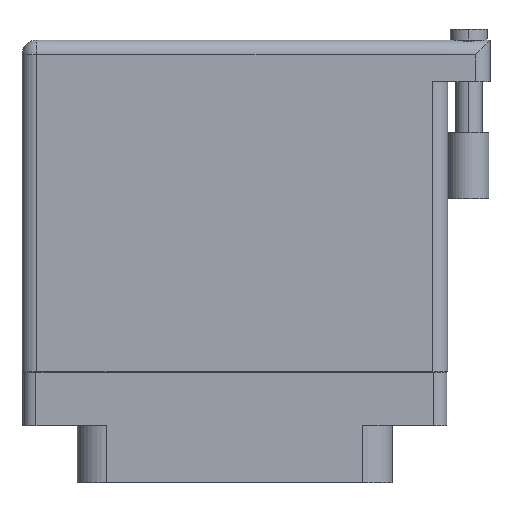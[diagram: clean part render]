
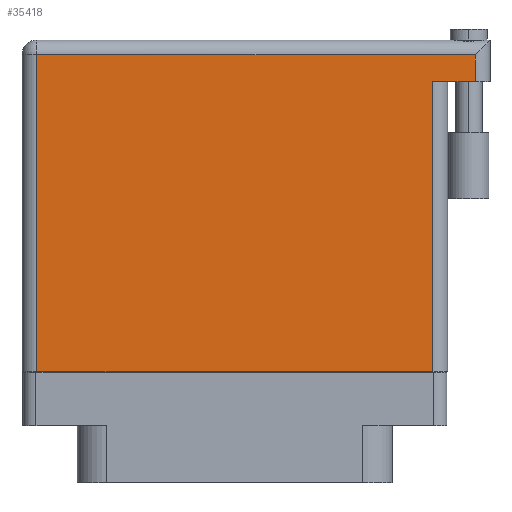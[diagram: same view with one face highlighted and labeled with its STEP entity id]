
A CAD part, front view. The second image highlights one B-rep face of the part: STEP entity #35418.
In plain terms, the highlighted face is planar.
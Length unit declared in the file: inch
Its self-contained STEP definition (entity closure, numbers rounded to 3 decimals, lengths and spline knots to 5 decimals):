
#506 = EDGE_CURVE ( 'NONE', #37140, #34961, #4797, .T. ) ;
#1290 = EDGE_CURVE ( 'NONE', #16771, #7316, #10068, .T. ) ;
#1339 = LINE ( 'NONE', #14774, #28770 ) ;
#1908 = CARTESIAN_POINT ( 'NONE',  ( 0.934, 1.269, 0.4495 ) ) ;
#2049 = DIRECTION ( 'NONE',  ( -1., 0., 0. ) ) ;
#2060 = EDGE_CURVE ( 'NONE', #34961, #11494, #1339, .T. ) ;
#2400 = PLANE ( 'NONE',  #3954 ) ;
#2405 = DIRECTION ( 'NONE',  ( 0., -1., 0. ) ) ;
#3937 = VECTOR ( 'NONE', #26450, 39.37008 ) ;
#3954 = AXIS2_PLACEMENT_3D ( 'NONE', #21040, #33476, #18112 ) ;
#4003 = CARTESIAN_POINT ( 'NONE',  ( 1.134, 1.466, 0.4495 ) ) ;
#4797 = LINE ( 'NONE', #32863, #17341 ) ;
#5541 = EDGE_CURVE ( 'NONE', #11494, #21737, #5852, .T. ) ;
#5654 = ORIENTED_EDGE ( 'NONE', *, *, #12906, .T. ) ;
#5807 = EDGE_LOOP ( 'NONE', ( #34716, #5654, #22525, #21060, #19671, #14708 ) ) ;
#5836 = DIRECTION ( 'NONE',  ( 1., 0., 0. ) ) ;
#5852 = LINE ( 'NONE', #18614, #23176 ) ;
#6847 = CARTESIAN_POINT ( 'NONE',  ( 0.934, -0.1, 0.4495 ) ) ;
#7316 = VERTEX_POINT ( 'NONE', #39706 ) ;
#7902 = FACE_OUTER_BOUND ( 'NONE', #5807, .T. ) ;
#9822 = DIRECTION ( 'NONE',  ( -1., 0., 0. ) ) ;
#10068 = LINE ( 'NONE', #12647, #31269 ) ;
#11494 = VERTEX_POINT ( 'NONE', #35452 ) ;
#12647 = CARTESIAN_POINT ( 'NONE',  ( 1.204, 1.269, 0.4495 ) ) ;
#12906 = EDGE_CURVE ( 'NONE', #21737, #7316, #27032, .T. ) ;
#13142 = LINE ( 'NONE', #4003, #30462 ) ;
#14708 = ORIENTED_EDGE ( 'NONE', *, *, #2060, .T. ) ;
#14774 = CARTESIAN_POINT ( 'NONE',  ( -0.934, -0.1, 0.4495 ) ) ;
#15809 = CARTESIAN_POINT ( 'NONE',  ( 1.134, 1.269, 0.4495 ) ) ;
#16771 = VERTEX_POINT ( 'NONE', #15809 ) ;
#17341 = VECTOR ( 'NONE', #2049, 39.37008 ) ;
#18112 = DIRECTION ( 'NONE',  ( -1., 0., 0. ) ) ;
#18614 = CARTESIAN_POINT ( 'NONE',  ( -1.004, -0.1, 0.4495 ) ) ;
#19198 = DIRECTION ( 'NONE',  ( 0., 1., 0. ) ) ;
#19671 = ORIENTED_EDGE ( 'NONE', *, *, #506, .T. ) ;
#21040 = CARTESIAN_POINT ( 'NONE',  ( -1.004, 1.466, 0.4495 ) ) ;
#21060 = ORIENTED_EDGE ( 'NONE', *, *, #26642, .T. ) ;
#21737 = VERTEX_POINT ( 'NONE', #6847 ) ;
#22280 = CARTESIAN_POINT ( 'NONE',  ( -0.934, 1.396, 0.4495 ) ) ;
#22525 = ORIENTED_EDGE ( 'NONE', *, *, #1290, .F. ) ;
#23176 = VECTOR ( 'NONE', #5836, 39.37008 ) ;
#25771 = CARTESIAN_POINT ( 'NONE',  ( 1.134, 1.396, 0.4495 ) ) ;
#26450 = DIRECTION ( 'NONE',  ( 0., 1., 0. ) ) ;
#26642 = EDGE_CURVE ( 'NONE', #16771, #37140, #13142, .T. ) ;
#27032 = LINE ( 'NONE', #1908, #3937 ) ;
#28770 = VECTOR ( 'NONE', #2405, 39.37008 ) ;
#30462 = VECTOR ( 'NONE', #19198, 39.37008 ) ;
#31269 = VECTOR ( 'NONE', #9822, 39.37008 ) ;
#32863 = CARTESIAN_POINT ( 'NONE',  ( -1.004, 1.396, 0.4495 ) ) ;
#33476 = DIRECTION ( 'NONE',  ( 0., 0., -1. ) ) ;
#34716 = ORIENTED_EDGE ( 'NONE', *, *, #5541, .T. ) ;
#34961 = VERTEX_POINT ( 'NONE', #22280 ) ;
#35418 = ADVANCED_FACE ( 'NONE', ( #7902 ), #2400, .F. ) ;
#35452 = CARTESIAN_POINT ( 'NONE',  ( -0.934, -0.1, 0.4495 ) ) ;
#37140 = VERTEX_POINT ( 'NONE', #25771 ) ;
#39706 = CARTESIAN_POINT ( 'NONE',  ( 0.934, 1.269, 0.4495 ) ) ;
